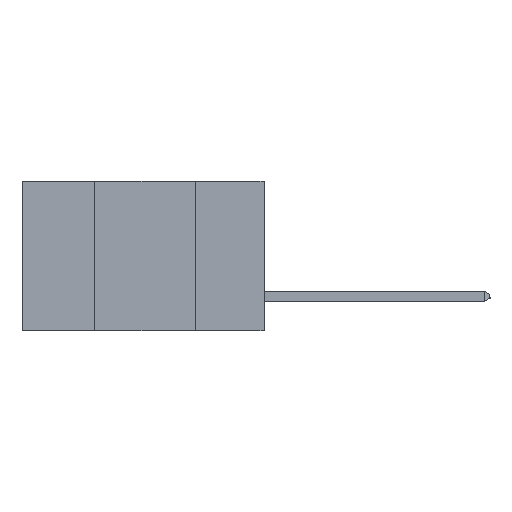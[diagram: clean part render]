
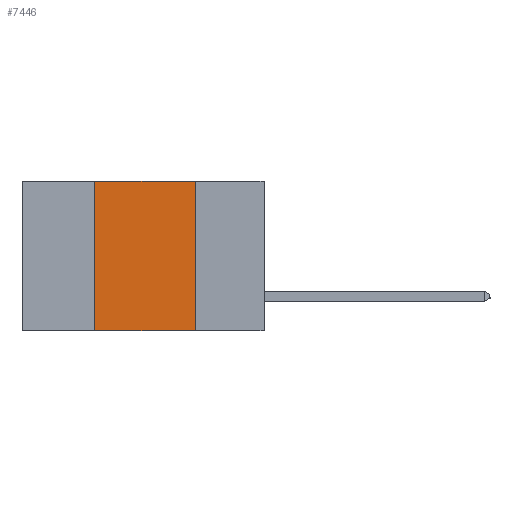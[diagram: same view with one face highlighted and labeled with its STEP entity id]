
A CAD part, left-side view. The second image highlights one B-rep face of the part: STEP entity #7446.
In plain terms, the highlighted planar face has unit normal (-1, 0, 0).
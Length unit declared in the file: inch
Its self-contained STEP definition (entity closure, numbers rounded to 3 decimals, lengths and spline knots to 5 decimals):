
#489 = CARTESIAN_POINT ( 'NONE',  ( 0., 0.42, 0. ) ) ;
#1141 = FACE_OUTER_BOUND ( 'NONE', #10608, .T. ) ;
#1386 = AXIS2_PLACEMENT_3D ( 'NONE', #3443, #6273, #3239 ) ;
#1390 = CARTESIAN_POINT ( 'NONE',  ( 0., 0.6, -0.37 ) ) ;
#1595 = ORIENTED_EDGE ( 'NONE', *, *, #9751, .F. ) ;
#1627 = VERTEX_POINT ( 'NONE', #13744 ) ;
#2001 = DIRECTION ( 'NONE',  ( 0., 0., 1. ) ) ;
#2014 = ORIENTED_EDGE ( 'NONE', *, *, #14848, .F. ) ;
#2976 = LINE ( 'NONE', #10995, #12795 ) ;
#3016 = VERTEX_POINT ( 'NONE', #489 ) ;
#3239 = DIRECTION ( 'NONE',  ( 0., 0., -1. ) ) ;
#3443 = CARTESIAN_POINT ( 'NONE',  ( 0., 0.6, 0. ) ) ;
#3606 = EDGE_CURVE ( 'NONE', #3016, #1627, #12526, .T. ) ;
#4672 = PLANE ( 'NONE',  #1386 ) ;
#4818 = CARTESIAN_POINT ( 'NONE',  ( 0., 0.17, 0. ) ) ;
#5149 = LINE ( 'NONE', #4818, #14525 ) ;
#6273 = DIRECTION ( 'NONE',  ( 1., 0., 0. ) ) ;
#7434 = DIRECTION ( 'NONE',  ( 0., 0., -1. ) ) ;
#7446 = ADVANCED_FACE ( 'NONE', ( #1141 ), #4672, .F. ) ;
#7943 = DIRECTION ( 'NONE',  ( 0., -1., 0. ) ) ;
#8352 = CARTESIAN_POINT ( 'NONE',  ( 0., 0.6, 0. ) ) ;
#8392 = DIRECTION ( 'NONE',  ( 0., -1., 0. ) ) ;
#9674 = VERTEX_POINT ( 'NONE', #11025 ) ;
#9751 = EDGE_CURVE ( 'NONE', #1627, #9674, #5149, .T. ) ;
#10608 = EDGE_LOOP ( 'NONE', ( #1595, #15253, #2014, #12661 ) ) ;
#10995 = CARTESIAN_POINT ( 'NONE',  ( 0., 0.42, 0. ) ) ;
#11025 = CARTESIAN_POINT ( 'NONE',  ( 0., 0.17, -0.37 ) ) ;
#12526 = LINE ( 'NONE', #8352, #15911 ) ;
#12661 = ORIENTED_EDGE ( 'NONE', *, *, #15704, .T. ) ;
#12767 = VECTOR ( 'NONE', #7943, 39.37008 ) ;
#12795 = VECTOR ( 'NONE', #2001, 39.37008 ) ;
#13744 = CARTESIAN_POINT ( 'NONE',  ( 0., 0.17, 0. ) ) ;
#14389 = VERTEX_POINT ( 'NONE', #15067 ) ;
#14525 = VECTOR ( 'NONE', #7434, 39.37008 ) ;
#14848 = EDGE_CURVE ( 'NONE', #14389, #3016, #2976, .T. ) ;
#15067 = CARTESIAN_POINT ( 'NONE',  ( 0., 0.42, -0.37 ) ) ;
#15253 = ORIENTED_EDGE ( 'NONE', *, *, #3606, .F. ) ;
#15704 = EDGE_CURVE ( 'NONE', #14389, #9674, #16151, .T. ) ;
#15911 = VECTOR ( 'NONE', #8392, 39.37008 ) ;
#16151 = LINE ( 'NONE', #1390, #12767 ) ;
